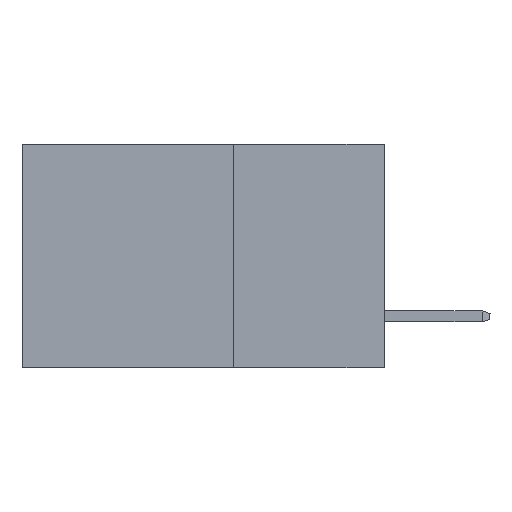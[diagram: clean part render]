
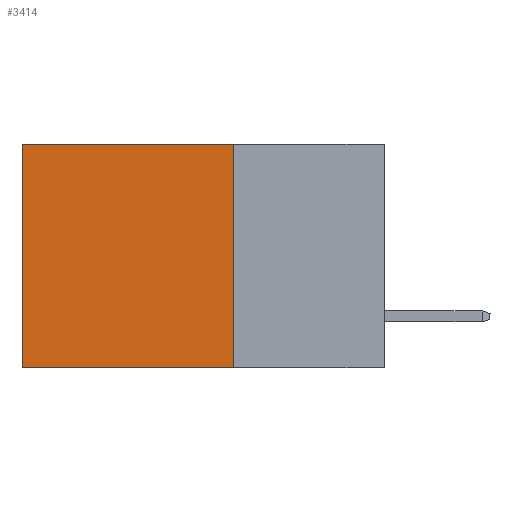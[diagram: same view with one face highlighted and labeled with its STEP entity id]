
A CAD part, left-side view. The second image highlights one B-rep face of the part: STEP entity #3414.
In plain terms, the highlighted planar face has unit normal (-1, 0, 0).
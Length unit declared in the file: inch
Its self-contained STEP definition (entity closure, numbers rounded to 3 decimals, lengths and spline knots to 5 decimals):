
#818 = DIRECTION ( 'NONE',  ( 0., 0., -1. ) ) ;
#1567 = VERTEX_POINT ( 'NONE', #3294 ) ;
#1855 = ORIENTED_EDGE ( 'NONE', *, *, #5743, .F. ) ;
#2068 = ORIENTED_EDGE ( 'NONE', *, *, #15959, .T. ) ;
#2171 = CARTESIAN_POINT ( 'NONE',  ( 0.2615, 0.25, -0.37 ) ) ;
#2217 = DIRECTION ( 'NONE',  ( 0., 0., -1. ) ) ;
#2773 = LINE ( 'NONE', #12810, #14140 ) ;
#3176 = VECTOR ( 'NONE', #3722, 39.37008 ) ;
#3294 = CARTESIAN_POINT ( 'NONE',  ( 0.2615, 0.6, 0. ) ) ;
#3414 = ADVANCED_FACE ( 'NONE', ( #7091 ), #15728, .F. ) ;
#3722 = DIRECTION ( 'NONE',  ( 0., 1., 0. ) ) ;
#4377 = EDGE_CURVE ( 'NONE', #10228, #9053, #13498, .T. ) ;
#4415 = DIRECTION ( 'NONE',  ( 1., 0., 0. ) ) ;
#5743 = EDGE_CURVE ( 'NONE', #11859, #10228, #9536, .T. ) ;
#6016 = VECTOR ( 'NONE', #14480, 39.37008 ) ;
#6372 = DIRECTION ( 'NONE',  ( 0., 1., 0. ) ) ;
#7091 = FACE_OUTER_BOUND ( 'NONE', #8937, .T. ) ;
#7549 = ORIENTED_EDGE ( 'NONE', *, *, #4377, .F. ) ;
#8185 = EDGE_CURVE ( 'NONE', #11859, #1567, #2773, .T. ) ;
#8244 = AXIS2_PLACEMENT_3D ( 'NONE', #10693, #4415, #818 ) ;
#8526 = CARTESIAN_POINT ( 'NONE',  ( 0.2615, 0.25, -0.37 ) ) ;
#8937 = EDGE_LOOP ( 'NONE', ( #2068, #7549, #1855, #15506 ) ) ;
#9053 = VERTEX_POINT ( 'NONE', #13191 ) ;
#9536 = LINE ( 'NONE', #2171, #6016 ) ;
#9581 = CARTESIAN_POINT ( 'NONE',  ( 0.2615, 0.25, 0. ) ) ;
#10228 = VERTEX_POINT ( 'NONE', #15213 ) ;
#10693 = CARTESIAN_POINT ( 'NONE',  ( 0.2615, 0.25, -0.37 ) ) ;
#11859 = VERTEX_POINT ( 'NONE', #9581 ) ;
#12203 = VECTOR ( 'NONE', #2217, 39.37008 ) ;
#12810 = CARTESIAN_POINT ( 'NONE',  ( 0.2615, 0.25, 0. ) ) ;
#13191 = CARTESIAN_POINT ( 'NONE',  ( 0.2615, 0.6, -0.37 ) ) ;
#13321 = LINE ( 'NONE', #15837, #12203 ) ;
#13498 = LINE ( 'NONE', #8526, #3176 ) ;
#14140 = VECTOR ( 'NONE', #6372, 39.37008 ) ;
#14480 = DIRECTION ( 'NONE',  ( 0., 0., -1. ) ) ;
#15213 = CARTESIAN_POINT ( 'NONE',  ( 0.2615, 0.25, -0.37 ) ) ;
#15506 = ORIENTED_EDGE ( 'NONE', *, *, #8185, .T. ) ;
#15728 = PLANE ( 'NONE',  #8244 ) ;
#15837 = CARTESIAN_POINT ( 'NONE',  ( 0.2615, 0.6, -0.37 ) ) ;
#15959 = EDGE_CURVE ( 'NONE', #1567, #9053, #13321, .T. ) ;
